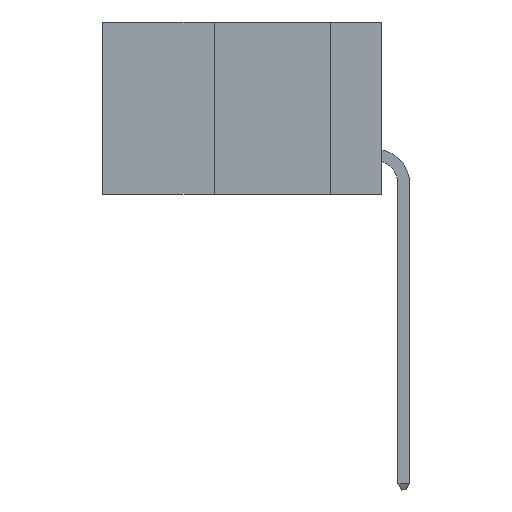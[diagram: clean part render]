
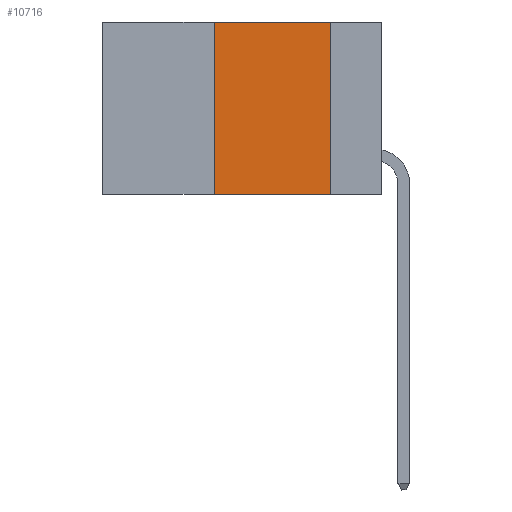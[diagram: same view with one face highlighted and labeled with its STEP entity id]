
A CAD part, left-side view. The second image highlights one B-rep face of the part: STEP entity #10716.
In plain terms, the highlighted planar face has unit normal (-1, 0, 0).
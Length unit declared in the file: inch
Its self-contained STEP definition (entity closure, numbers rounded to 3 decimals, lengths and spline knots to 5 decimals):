
#1407 = EDGE_LOOP ( 'NONE', ( #12818, #2959, #11227, #1412 ) ) ;
#1412 = ORIENTED_EDGE ( 'NONE', *, *, #8969, .T. ) ;
#1791 = AXIS2_PLACEMENT_3D ( 'NONE', #11865, #4354, #13030 ) ;
#1994 = CARTESIAN_POINT ( 'NONE',  ( 0., 0.11, -0.37 ) ) ;
#2698 = DIRECTION ( 'NONE',  ( 0., 0., 1. ) ) ;
#2959 = ORIENTED_EDGE ( 'NONE', *, *, #7638, .F. ) ;
#3141 = LINE ( 'NONE', #4268, #7448 ) ;
#3205 = FACE_OUTER_BOUND ( 'NONE', #1407, .T. ) ;
#3437 = LINE ( 'NONE', #9741, #5704 ) ;
#3602 = CARTESIAN_POINT ( 'NONE',  ( 0., 0.36, 0. ) ) ;
#4268 = CARTESIAN_POINT ( 'NONE',  ( 0., 0.6, 0. ) ) ;
#4354 = DIRECTION ( 'NONE',  ( 1., 0., 0. ) ) ;
#4755 = CARTESIAN_POINT ( 'NONE',  ( 0., 0.11, 0. ) ) ;
#4898 = DIRECTION ( 'NONE',  ( 0., 0., -1. ) ) ;
#5526 = CARTESIAN_POINT ( 'NONE',  ( 0., 0.11, 0. ) ) ;
#5622 = PLANE ( 'NONE',  #1791 ) ;
#5704 = VECTOR ( 'NONE', #10720, 39.37008 ) ;
#6062 = VERTEX_POINT ( 'NONE', #11787 ) ;
#6902 = VECTOR ( 'NONE', #2698, 39.37008 ) ;
#7314 = EDGE_CURVE ( 'NONE', #8975, #7812, #10035, .T. ) ;
#7448 = VECTOR ( 'NONE', #10276, 39.37008 ) ;
#7638 = EDGE_CURVE ( 'NONE', #9714, #8975, #3141, .T. ) ;
#7812 = VERTEX_POINT ( 'NONE', #1994 ) ;
#8831 = LINE ( 'NONE', #3602, #6902 ) ;
#8969 = EDGE_CURVE ( 'NONE', #6062, #7812, #3437, .T. ) ;
#8975 = VERTEX_POINT ( 'NONE', #4755 ) ;
#9418 = CARTESIAN_POINT ( 'NONE',  ( 0., 0.36, 0. ) ) ;
#9714 = VERTEX_POINT ( 'NONE', #9418 ) ;
#9741 = CARTESIAN_POINT ( 'NONE',  ( 0., 0.6, -0.37 ) ) ;
#10035 = LINE ( 'NONE', #5526, #10330 ) ;
#10276 = DIRECTION ( 'NONE',  ( 0., -1., 0. ) ) ;
#10330 = VECTOR ( 'NONE', #4898, 39.37008 ) ;
#10412 = EDGE_CURVE ( 'NONE', #6062, #9714, #8831, .T. ) ;
#10716 = ADVANCED_FACE ( 'NONE', ( #3205 ), #5622, .F. ) ;
#10720 = DIRECTION ( 'NONE',  ( 0., -1., 0. ) ) ;
#11227 = ORIENTED_EDGE ( 'NONE', *, *, #10412, .F. ) ;
#11787 = CARTESIAN_POINT ( 'NONE',  ( 0., 0.36, -0.37 ) ) ;
#11865 = CARTESIAN_POINT ( 'NONE',  ( 0., 0.6, 0. ) ) ;
#12818 = ORIENTED_EDGE ( 'NONE', *, *, #7314, .F. ) ;
#13030 = DIRECTION ( 'NONE',  ( 0., 0., -1. ) ) ;
